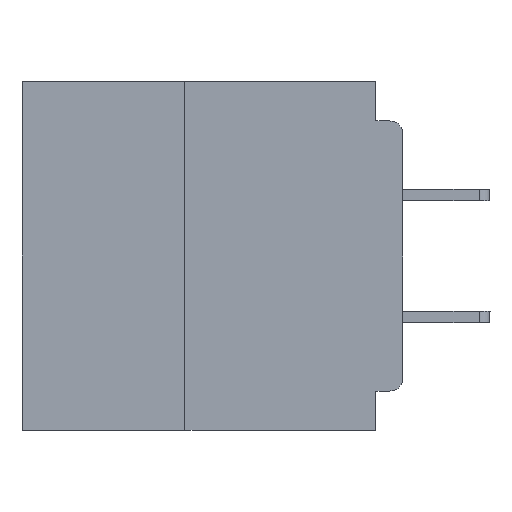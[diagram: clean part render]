
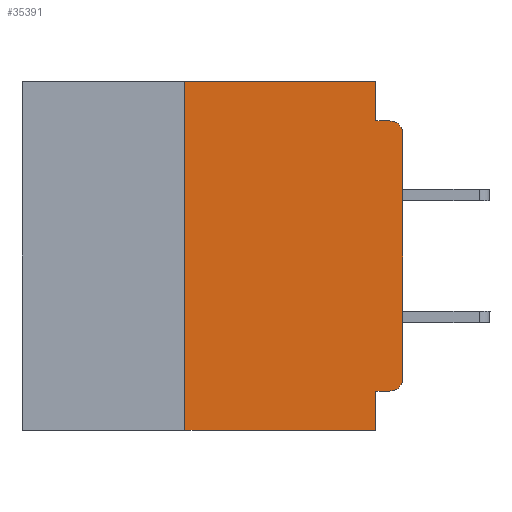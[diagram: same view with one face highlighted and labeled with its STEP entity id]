
A CAD part, left-side view. The second image highlights one B-rep face of the part: STEP entity #35391.
In plain terms, the highlighted planar face has unit normal (-1, 0, 0).
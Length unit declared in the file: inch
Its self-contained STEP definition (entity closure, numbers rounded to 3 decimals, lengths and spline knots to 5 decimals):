
#52 = VERTEX_POINT ( 'NONE', #8151 ) ;
#663 = DIRECTION ( 'NONE',  ( 0., 1., 0. ) ) ;
#1075 = AXIS2_PLACEMENT_3D ( 'NONE', #4275, #18968, #52750 ) ;
#1429 = CARTESIAN_POINT ( 'NONE',  ( 0., 0., -0.06 ) ) ;
#1765 = CARTESIAN_POINT ( 'NONE',  ( 0., 0.437, -0.4 ) ) ;
#2063 = FACE_OUTER_BOUND ( 'NONE', #56833, .T. ) ;
#3479 = DIRECTION ( 'NONE',  ( 0., -1., 0. ) ) ;
#4275 = CARTESIAN_POINT ( 'NONE',  ( 0., 0.437, 0. ) ) ;
#5538 = ORIENTED_EDGE ( 'NONE', *, *, #32403, .T. ) ;
#6836 = EDGE_CURVE ( 'NONE', #17005, #52, #44328, .T. ) ;
#7596 = VECTOR ( 'NONE', #21331, 39.37008 ) ;
#8151 = CARTESIAN_POINT ( 'NONE',  ( 0., 0.031, -0.355 ) ) ;
#8263 = ORIENTED_EDGE ( 'NONE', *, *, #10347, .F. ) ;
#8445 = VECTOR ( 'NONE', #3479, 39.37008 ) ;
#9131 = LINE ( 'NONE', #55057, #7596 ) ;
#9235 = VECTOR ( 'NONE', #16491, 39.37008 ) ;
#9857 = CARTESIAN_POINT ( 'NONE',  ( 0., 0.25, -0.4 ) ) ;
#10161 = CARTESIAN_POINT ( 'NONE',  ( 0., 0., -0.34 ) ) ;
#10347 = EDGE_CURVE ( 'NONE', #60521, #51120, #38175, .T. ) ;
#10421 = AXIS2_PLACEMENT_3D ( 'NONE', #54339, #25444, #59142 ) ;
#13443 = VECTOR ( 'NONE', #33112, 39.37008 ) ;
#14087 = PLANE ( 'NONE',  #1075 ) ;
#16287 = EDGE_CURVE ( 'NONE', #54992, #51120, #60122, .T. ) ;
#16491 = DIRECTION ( 'NONE',  ( 0., -1., 0. ) ) ;
#16913 = LINE ( 'NONE', #35475, #28263 ) ;
#17005 = VERTEX_POINT ( 'NONE', #49769 ) ;
#18624 = VECTOR ( 'NONE', #663, 39.37008 ) ;
#18968 = DIRECTION ( 'NONE',  ( 1., 0., 0. ) ) ;
#19978 = ORIENTED_EDGE ( 'NONE', *, *, #6836, .F. ) ;
#21331 = DIRECTION ( 'NONE',  ( 0., 0., -1. ) ) ;
#21399 = LINE ( 'NONE', #61382, #8445 ) ;
#21448 = ORIENTED_EDGE ( 'NONE', *, *, #26718, .F. ) ;
#21667 = CARTESIAN_POINT ( 'NONE',  ( 0., 0., -0.045 ) ) ;
#25416 = VERTEX_POINT ( 'NONE', #47701 ) ;
#25444 = DIRECTION ( 'NONE',  ( -1., 0., 0. ) ) ;
#26077 = DIRECTION ( 'NONE',  ( -1., 0., 0. ) ) ;
#26718 = EDGE_CURVE ( 'NONE', #52, #42093, #9131, .T. ) ;
#27833 = VERTEX_POINT ( 'NONE', #10161 ) ;
#27986 = ORIENTED_EDGE ( 'NONE', *, *, #16287, .T. ) ;
#28245 = CARTESIAN_POINT ( 'NONE',  ( 0., 0.25, -0.4 ) ) ;
#28263 = VECTOR ( 'NONE', #40278, 39.37008 ) ;
#28545 = CARTESIAN_POINT ( 'NONE',  ( 0., 0.25, 0. ) ) ;
#31531 = VERTEX_POINT ( 'NONE', #9857 ) ;
#31725 = EDGE_CURVE ( 'NONE', #27833, #54992, #16913, .T. ) ;
#32403 = EDGE_CURVE ( 'NONE', #17005, #27833, #51584, .T. ) ;
#33112 = DIRECTION ( 'NONE',  ( 0., 0., 1. ) ) ;
#34043 = VECTOR ( 'NONE', #51371, 39.37008 ) ;
#35391 = ADVANCED_FACE ( 'NONE', ( #2063 ), #14087, .F. ) ;
#35475 = CARTESIAN_POINT ( 'NONE',  ( 0., 0., 0. ) ) ;
#36670 = VECTOR ( 'NONE', #50564, 39.37008 ) ;
#38175 = LINE ( 'NONE', #21667, #36670 ) ;
#38793 = CARTESIAN_POINT ( 'NONE',  ( 0., 0.031, -0.4 ) ) ;
#38942 = EDGE_CURVE ( 'NONE', #54035, #25416, #21399, .T. ) ;
#39141 = LINE ( 'NONE', #28245, #13443 ) ;
#39585 = CARTESIAN_POINT ( 'NONE',  ( 0., 0.015, -0.045 ) ) ;
#40278 = DIRECTION ( 'NONE',  ( 0., 0., 1. ) ) ;
#40387 = AXIS2_PLACEMENT_3D ( 'NONE', #54969, #26077, #59792 ) ;
#41179 = EDGE_CURVE ( 'NONE', #25416, #60521, #46862, .T. ) ;
#42093 = VERTEX_POINT ( 'NONE', #38793 ) ;
#44328 = LINE ( 'NONE', #44361, #18624 ) ;
#44361 = CARTESIAN_POINT ( 'NONE',  ( 0., 0., -0.355 ) ) ;
#46514 = CARTESIAN_POINT ( 'NONE',  ( 0., 0.031, 0. ) ) ;
#46862 = LINE ( 'NONE', #46514, #34043 ) ;
#47205 = EDGE_CURVE ( 'NONE', #31531, #42093, #60582, .T. ) ;
#47671 = ORIENTED_EDGE ( 'NONE', *, *, #38942, .F. ) ;
#47701 = CARTESIAN_POINT ( 'NONE',  ( 0., 0.031, 0. ) ) ;
#49769 = CARTESIAN_POINT ( 'NONE',  ( 0., 0.015, -0.355 ) ) ;
#50564 = DIRECTION ( 'NONE',  ( 0., -1., 0. ) ) ;
#51120 = VERTEX_POINT ( 'NONE', #39585 ) ;
#51371 = DIRECTION ( 'NONE',  ( 0., 0., -1. ) ) ;
#51422 = ORIENTED_EDGE ( 'NONE', *, *, #41179, .F. ) ;
#51584 = CIRCLE ( 'NONE', #40387, 0.015 ) ;
#52750 = DIRECTION ( 'NONE',  ( 0., 0., -1. ) ) ;
#53698 = ORIENTED_EDGE ( 'NONE', *, *, #54656, .F. ) ;
#54035 = VERTEX_POINT ( 'NONE', #28545 ) ;
#54339 = CARTESIAN_POINT ( 'NONE',  ( 0., 0.015, -0.06 ) ) ;
#54365 = ORIENTED_EDGE ( 'NONE', *, *, #31725, .T. ) ;
#54656 = EDGE_CURVE ( 'NONE', #31531, #54035, #39141, .T. ) ;
#54969 = CARTESIAN_POINT ( 'NONE',  ( 0., 0.015, -0.34 ) ) ;
#54992 = VERTEX_POINT ( 'NONE', #1429 ) ;
#55057 = CARTESIAN_POINT ( 'NONE',  ( 0., 0.031, -0.4 ) ) ;
#55317 = ORIENTED_EDGE ( 'NONE', *, *, #47205, .T. ) ;
#56833 = EDGE_LOOP ( 'NONE', ( #54365, #27986, #8263, #51422, #47671, #53698, #55317, #21448, #19978, #5538 ) ) ;
#59142 = DIRECTION ( 'NONE',  ( 0., 0., -1. ) ) ;
#59792 = DIRECTION ( 'NONE',  ( 0., 0., -1. ) ) ;
#60122 = CIRCLE ( 'NONE', #10421, 0.015 ) ;
#60521 = VERTEX_POINT ( 'NONE', #61634 ) ;
#60582 = LINE ( 'NONE', #1765, #9235 ) ;
#61382 = CARTESIAN_POINT ( 'NONE',  ( 0., 0.437, 0. ) ) ;
#61634 = CARTESIAN_POINT ( 'NONE',  ( 0., 0.031, -0.045 ) ) ;
